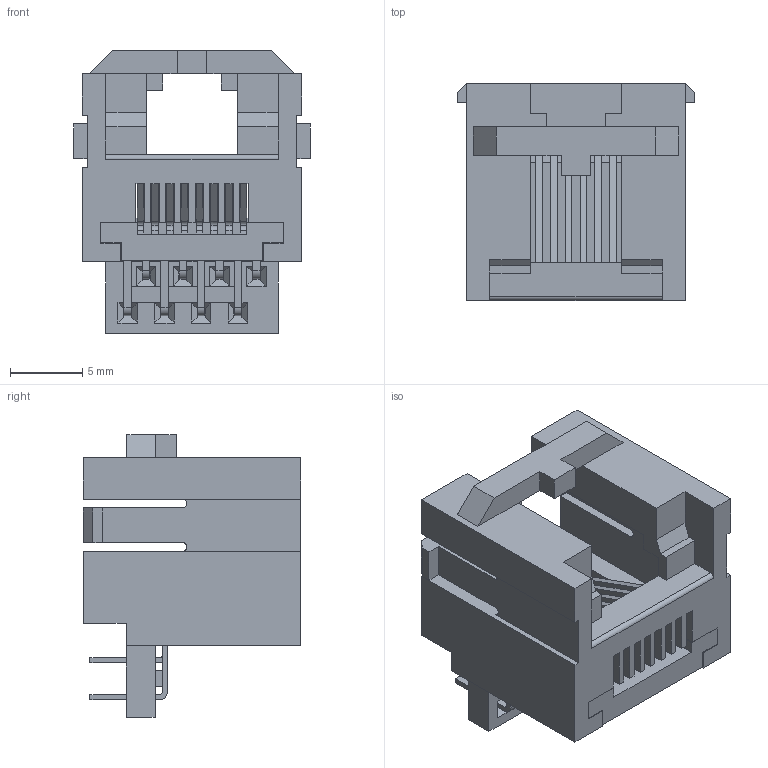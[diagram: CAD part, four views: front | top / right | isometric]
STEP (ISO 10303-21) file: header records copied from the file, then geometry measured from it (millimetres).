
FILE_DESCRIPTION (( 'STEP AP203' ), '1' );
FILE_NAME ('JPG018836P00035.STEP', '2020-03-17T19:05:36', ( '' ), ( '' ), 'SwSTEP 2.0', 'SolidWorks 2016', '' );
FILE_SCHEMA (( 'CONFIG_CONTROL_DESIGN' ));
Length unit declared in the file: millimetre
Products named in the file (4): PG Contact Lock; JPG018836P00035; PG Contacts; PG Insulator
Assembly tree (3 placements, depth 2):
  JPG018836P00035
    PG Insulator
    PG Contacts
    PG Contact Lock
Bounding box: 16.35 x 15 x 19.55 mm (x, y, z)
Volume: 1392 mm3; surface area: 2706.5 mm2
Topology: 10 solids, 10 shells, 542 faces, 1552 edges, 1012 vertices
Faces by surface type: plane 461, cylinder 69, bspline 12
Entity records: 18702 total; most frequent: CARTESIAN_POINT 4502, ORIENTED_EDGE 3104, DIRECTION 2455, EDGE_CURVE 1552, VECTOR 1347, LINE 1347, VERTEX_POINT 1012, EDGE_LOOP 560
